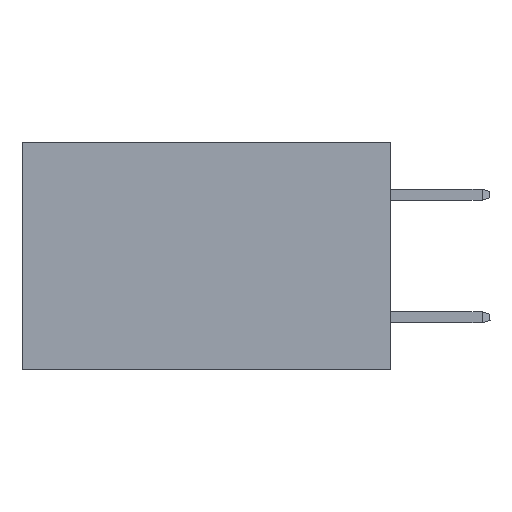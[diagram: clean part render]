
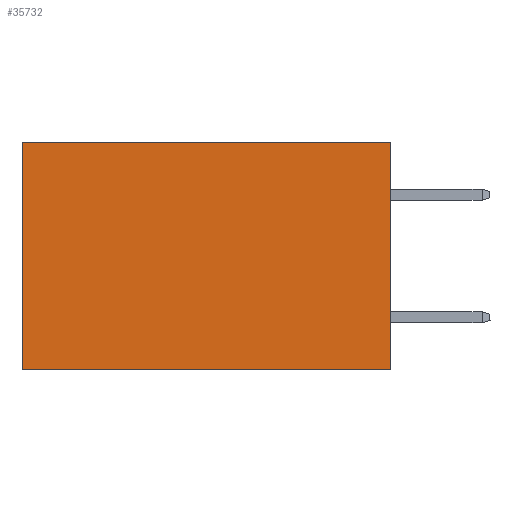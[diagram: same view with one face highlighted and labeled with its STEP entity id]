
A CAD part, left-side view. The second image highlights one B-rep face of the part: STEP entity #35732.
In plain terms, the highlighted planar face has unit normal (-1, 0, 0).
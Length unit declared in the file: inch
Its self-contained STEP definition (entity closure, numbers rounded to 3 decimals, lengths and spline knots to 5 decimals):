
#316 = ORIENTED_EDGE ( 'NONE', *, *, #28405, .T. ) ;
#757 = ORIENTED_EDGE ( 'NONE', *, *, #33569, .T. ) ;
#1398 = VERTEX_POINT ( 'NONE', #32781 ) ;
#4613 = DIRECTION ( 'NONE',  ( 0., 0., -1. ) ) ;
#4912 = VECTOR ( 'NONE', #19105, 39.37008 ) ;
#5006 = LINE ( 'NONE', #20312, #26283 ) ;
#5843 = CARTESIAN_POINT ( 'NONE',  ( 0.2875, 0., 0. ) ) ;
#6906 = VECTOR ( 'NONE', #4613, 39.37008 ) ;
#11700 = VERTEX_POINT ( 'NONE', #41794 ) ;
#12055 = DIRECTION ( 'NONE',  ( 1., 0., 0. ) ) ;
#14685 = EDGE_LOOP ( 'NONE', ( #316, #29771, #16432, #757 ) ) ;
#15236 = VERTEX_POINT ( 'NONE', #21135 ) ;
#16432 = ORIENTED_EDGE ( 'NONE', *, *, #34979, .F. ) ;
#16829 = CARTESIAN_POINT ( 'NONE',  ( 0.2875, 0., 0. ) ) ;
#18897 = DIRECTION ( 'NONE',  ( 0., 1., 0. ) ) ;
#19105 = DIRECTION ( 'NONE',  ( 0., 1., 0. ) ) ;
#19116 = LINE ( 'NONE', #16829, #4912 ) ;
#20312 = CARTESIAN_POINT ( 'NONE',  ( 0.2875, 0.6, 0. ) ) ;
#21135 = CARTESIAN_POINT ( 'NONE',  ( 0.2875, 0., 0. ) ) ;
#22000 = CARTESIAN_POINT ( 'NONE',  ( 0.2875, 0., -0.37 ) ) ;
#22110 = PLANE ( 'NONE',  #31616 ) ;
#23604 = DIRECTION ( 'NONE',  ( 0., 0., -1. ) ) ;
#24278 = LINE ( 'NONE', #22000, #41467 ) ;
#26283 = VECTOR ( 'NONE', #23604, 39.37008 ) ;
#27596 = LINE ( 'NONE', #40100, #6906 ) ;
#28405 = EDGE_CURVE ( 'NONE', #33061, #11700, #5006, .T. ) ;
#29771 = ORIENTED_EDGE ( 'NONE', *, *, #37591, .F. ) ;
#30068 = FACE_OUTER_BOUND ( 'NONE', #14685, .T. ) ;
#31616 = AXIS2_PLACEMENT_3D ( 'NONE', #5843, #12055, #37898 ) ;
#32781 = CARTESIAN_POINT ( 'NONE',  ( 0.2875, 0., -0.37 ) ) ;
#33061 = VERTEX_POINT ( 'NONE', #35526 ) ;
#33569 = EDGE_CURVE ( 'NONE', #15236, #33061, #19116, .T. ) ;
#34979 = EDGE_CURVE ( 'NONE', #15236, #1398, #27596, .T. ) ;
#35526 = CARTESIAN_POINT ( 'NONE',  ( 0.2875, 0.6, 0. ) ) ;
#35732 = ADVANCED_FACE ( 'NONE', ( #30068 ), #22110, .F. ) ;
#37591 = EDGE_CURVE ( 'NONE', #1398, #11700, #24278, .T. ) ;
#37898 = DIRECTION ( 'NONE',  ( 0., 0., -1. ) ) ;
#40100 = CARTESIAN_POINT ( 'NONE',  ( 0.2875, 0., 0. ) ) ;
#41467 = VECTOR ( 'NONE', #18897, 39.37008 ) ;
#41794 = CARTESIAN_POINT ( 'NONE',  ( 0.2875, 0.6, -0.37 ) ) ;
